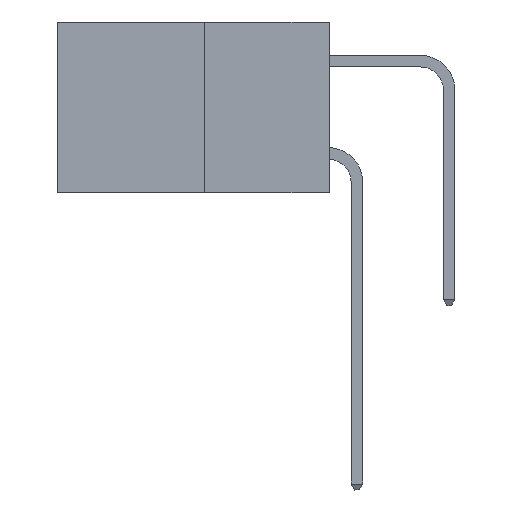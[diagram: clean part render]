
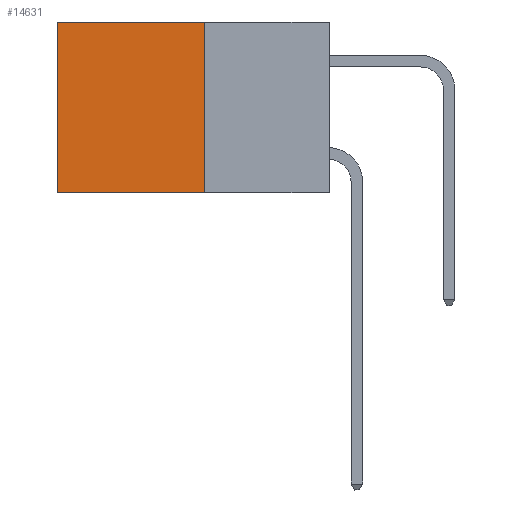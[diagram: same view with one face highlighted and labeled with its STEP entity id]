
A CAD part, left-side view. The second image highlights one B-rep face of the part: STEP entity #14631.
In plain terms, the highlighted planar face has unit normal (-1, 0, 0).
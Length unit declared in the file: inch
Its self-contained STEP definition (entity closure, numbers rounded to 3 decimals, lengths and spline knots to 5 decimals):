
#843 = CARTESIAN_POINT ( 'NONE',  ( 0.277, 0.27, 0. ) ) ;
#2595 = EDGE_CURVE ( 'NONE', #18118, #13727, #3402, .T. ) ;
#3023 = CARTESIAN_POINT ( 'NONE',  ( 0.277, 0.27, -0.37 ) ) ;
#3087 = VERTEX_POINT ( 'NONE', #13072 ) ;
#3121 = VERTEX_POINT ( 'NONE', #10027 ) ;
#3280 = VECTOR ( 'NONE', #19528, 39.37008 ) ;
#3402 = LINE ( 'NONE', #7345, #15806 ) ;
#4116 = CARTESIAN_POINT ( 'NONE',  ( 0.277, 0.59, 0. ) ) ;
#4714 = DIRECTION ( 'NONE',  ( 0., 0., -1. ) ) ;
#6216 = DIRECTION ( 'NONE',  ( 0., 0., -1. ) ) ;
#6275 = CARTESIAN_POINT ( 'NONE',  ( 0.277, 0.27, -0.37 ) ) ;
#6331 = PLANE ( 'NONE',  #11651 ) ;
#6451 = EDGE_LOOP ( 'NONE', ( #14185, #17099, #11273, #14774 ) ) ;
#6562 = DIRECTION ( 'NONE',  ( 0., 1., 0. ) ) ;
#7345 = CARTESIAN_POINT ( 'NONE',  ( 0.277, 0.27, 0. ) ) ;
#8631 = LINE ( 'NONE', #14572, #20588 ) ;
#10027 = CARTESIAN_POINT ( 'NONE',  ( 0.277, 0.27, -0.37 ) ) ;
#11273 = ORIENTED_EDGE ( 'NONE', *, *, #13512, .F. ) ;
#11651 = AXIS2_PLACEMENT_3D ( 'NONE', #3023, #14404, #4714 ) ;
#11829 = FACE_OUTER_BOUND ( 'NONE', #6451, .T. ) ;
#11849 = VECTOR ( 'NONE', #6216, 39.37008 ) ;
#12368 = LINE ( 'NONE', #6275, #11849 ) ;
#12577 = EDGE_CURVE ( 'NONE', #3121, #3087, #8631, .T. ) ;
#13072 = CARTESIAN_POINT ( 'NONE',  ( 0.277, 0.59, -0.37 ) ) ;
#13406 = CARTESIAN_POINT ( 'NONE',  ( 0.277, 0.59, -0.37 ) ) ;
#13512 = EDGE_CURVE ( 'NONE', #18118, #3121, #12368, .T. ) ;
#13727 = VERTEX_POINT ( 'NONE', #4116 ) ;
#14185 = ORIENTED_EDGE ( 'NONE', *, *, #16108, .T. ) ;
#14282 = DIRECTION ( 'NONE',  ( 0., 1., 0. ) ) ;
#14404 = DIRECTION ( 'NONE',  ( 1., 0., 0. ) ) ;
#14572 = CARTESIAN_POINT ( 'NONE',  ( 0.277, 0.27, -0.37 ) ) ;
#14631 = ADVANCED_FACE ( 'NONE', ( #11829 ), #6331, .F. ) ;
#14774 = ORIENTED_EDGE ( 'NONE', *, *, #2595, .T. ) ;
#15806 = VECTOR ( 'NONE', #6562, 39.37008 ) ;
#16108 = EDGE_CURVE ( 'NONE', #13727, #3087, #16165, .T. ) ;
#16165 = LINE ( 'NONE', #13406, #3280 ) ;
#17099 = ORIENTED_EDGE ( 'NONE', *, *, #12577, .F. ) ;
#18118 = VERTEX_POINT ( 'NONE', #843 ) ;
#19528 = DIRECTION ( 'NONE',  ( 0., 0., -1. ) ) ;
#20588 = VECTOR ( 'NONE', #14282, 39.37008 ) ;
